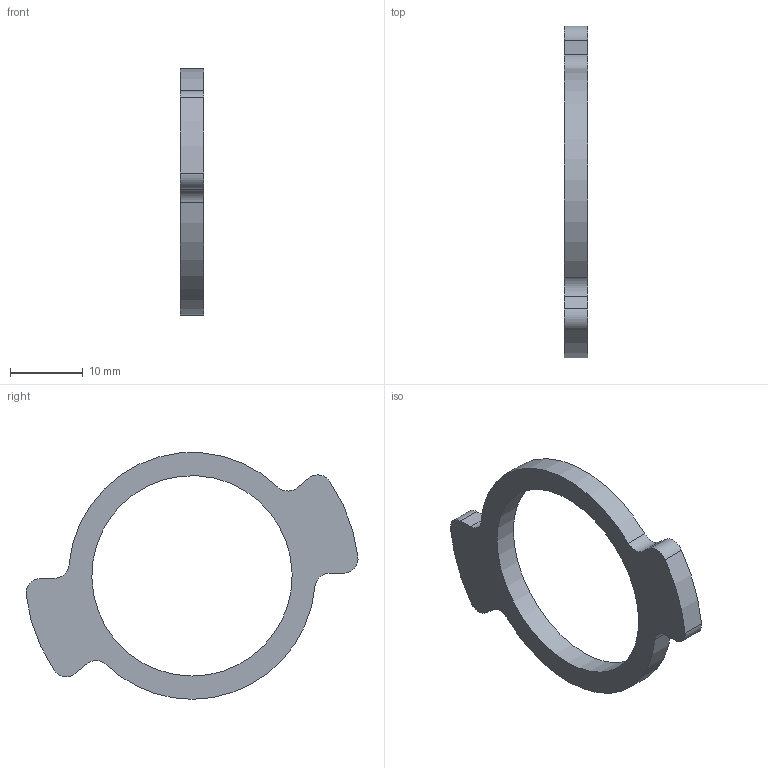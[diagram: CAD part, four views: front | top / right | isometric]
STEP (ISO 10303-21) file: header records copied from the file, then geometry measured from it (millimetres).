
FILE_DESCRIPTION(('FreeCAD Model'),'2;1');
FILE_NAME('Open CASCADE Shape Model','2022-06-07T14:30:38',('Author'),( ''),'Open CASCADE STEP processor 7.5','FreeCAD','Unknown');
FILE_SCHEMA(('AUTOMOTIVE_DESIGN { 1 0 10303 214 1 1 1 1 }'));
Length unit declared in the file: millimetre
Products named in the file (1): Locking Lug
Bounding box: 3.2 x 45.73 x 33.95 mm (x, y, z)
Volume: 1510.2 mm3; surface area: 1644.1 mm2
Topology: 1 solids, 1 shells, 19 faces, 61 edges, 44 vertices
Faces by surface type: cylinder 13, plane 6
Full cylindrical faces by diameter (mm): 27.6 x1
Entity records: 1584 total; most frequent: CARTESIAN_POINT 355, DIRECTION 241, ORIENTED_EDGE 122, PCURVE 122, DEFINITIONAL_REPRESENTATION 122, LINE 111, VECTOR 111, EDGE_CURVE 61
